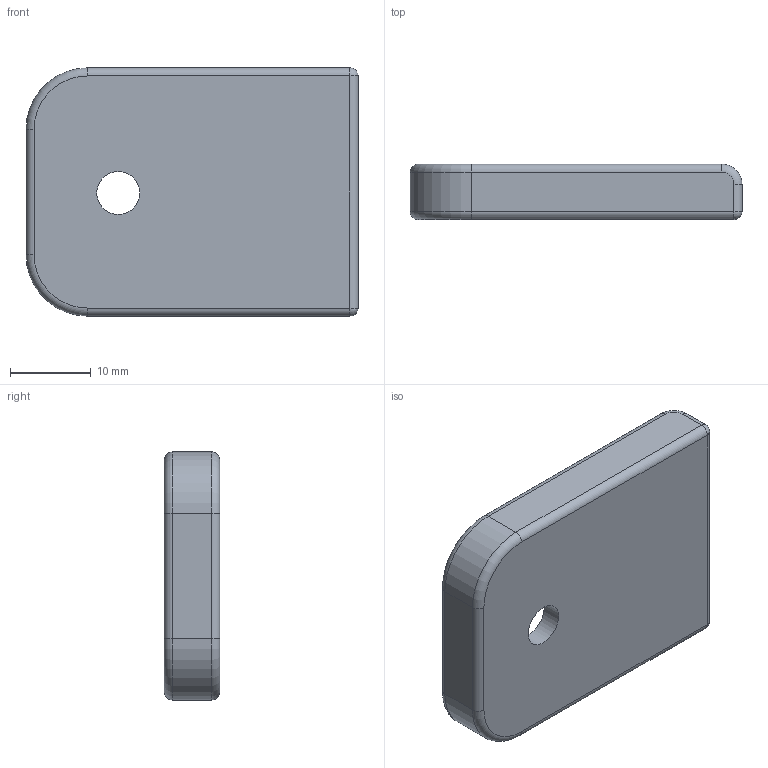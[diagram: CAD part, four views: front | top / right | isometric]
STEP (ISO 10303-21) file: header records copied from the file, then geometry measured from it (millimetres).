
FILE_DESCRIPTION(/* description */ (''),/* implementation_level */ '2;1');
FILE_NAME(/* name */ 'Glock Mag Baseplate v1.step',/* time_stamp */ '2019-08-25T22:27:07-04:00',/* author */ (''),/* organization */ (''),/* preprocessor_version */ 'ST-DEVELOPER v18',/* originating_system */ 'Autodesk Translation Framework v8.6.0.1094',/* authorisation */ '');
FILE_SCHEMA (('AUTOMOTIVE_DESIGN { 1 0 10303 214 3 1 1 }'));
Length unit declared in the file: millimetre
Products named in the file (1): Glock Mag Baseplate
Bounding box: 41.17 x 6.85 x 30.78 mm (x, y, z)
Volume: 4313.7 mm3; surface area: 3860.9 mm2
Topology: 1 solids, 1 shells, 59 faces, 149 edges, 92 vertices
Faces by surface type: plane 26, cylinder 23, torus 8, sphere 2
Full cylindrical faces by diameter (mm): 5.334 x1
Entity records: 1835 total; most frequent: CARTESIAN_POINT 323, DIRECTION 319, ORIENTED_EDGE 298, EDGE_CURVE 149, AXIS2_PLACEMENT_3D 112, LINE 95, VECTOR 95, VERTEX_POINT 92
